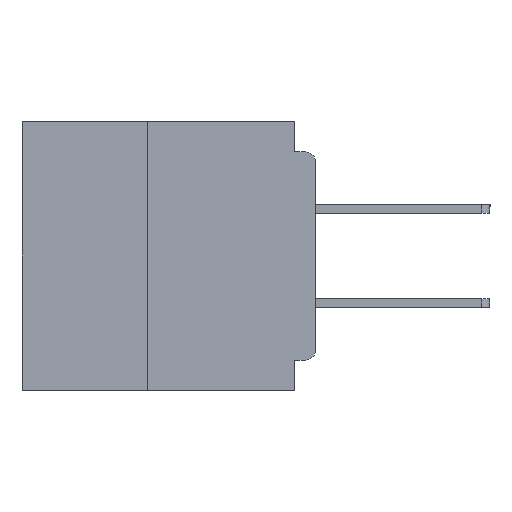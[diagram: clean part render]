
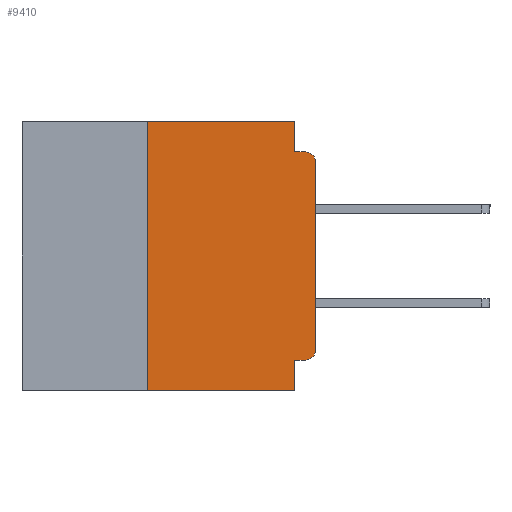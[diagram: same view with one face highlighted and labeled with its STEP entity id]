
A CAD part, left-side view. The second image highlights one B-rep face of the part: STEP entity #9410.
In plain terms, the highlighted planar face has unit normal (-1, 0, 0).
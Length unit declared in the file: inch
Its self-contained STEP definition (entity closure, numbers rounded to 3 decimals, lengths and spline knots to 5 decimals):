
#343 = VECTOR ( 'NONE', #35084, 39.37008 ) ;
#1396 = VECTOR ( 'NONE', #38408, 39.37008 ) ;
#1498 = VERTEX_POINT ( 'NONE', #6303 ) ;
#2432 = DIRECTION ( 'NONE',  ( 0., 0., -1. ) ) ;
#2590 = CARTESIAN_POINT ( 'NONE',  ( 0., 0.437, 0. ) ) ;
#2696 = EDGE_CURVE ( 'NONE', #32461, #8480, #12332, .T. ) ;
#3576 = CARTESIAN_POINT ( 'NONE',  ( 0., 0.031, 0. ) ) ;
#3684 = CARTESIAN_POINT ( 'NONE',  ( 0., 0.015, -0.06 ) ) ;
#4846 = CARTESIAN_POINT ( 'NONE',  ( 0., 0.437, -0.4 ) ) ;
#5216 = ORIENTED_EDGE ( 'NONE', *, *, #17932, .F. ) ;
#5430 = EDGE_CURVE ( 'NONE', #10705, #7421, #14539, .T. ) ;
#5847 = DIRECTION ( 'NONE',  ( 0., -1., 0. ) ) ;
#6114 = CARTESIAN_POINT ( 'NONE',  ( 0., 0.031, -0.4 ) ) ;
#6303 = CARTESIAN_POINT ( 'NONE',  ( 0., 0.25, -0.4 ) ) ;
#6957 = DIRECTION ( 'NONE',  ( 0., 0., -1. ) ) ;
#7421 = VERTEX_POINT ( 'NONE', #6114 ) ;
#7553 = CIRCLE ( 'NONE', #32367, 0.015 ) ;
#7854 = CARTESIAN_POINT ( 'NONE',  ( 0., 0.031, -0.045 ) ) ;
#8061 = CARTESIAN_POINT ( 'NONE',  ( 0., 0., -0.34 ) ) ;
#8124 = DIRECTION ( 'NONE',  ( 0., -1., 0. ) ) ;
#8434 = CARTESIAN_POINT ( 'NONE',  ( 0., 0.015, -0.34 ) ) ;
#8480 = VERTEX_POINT ( 'NONE', #8061 ) ;
#8983 = VECTOR ( 'NONE', #5847, 39.37008 ) ;
#9410 = ADVANCED_FACE ( 'NONE', ( #22653 ), #12601, .F. ) ;
#10026 = LINE ( 'NONE', #38281, #1396 ) ;
#10174 = VECTOR ( 'NONE', #24136, 39.37008 ) ;
#10698 = EDGE_CURVE ( 'NONE', #32712, #36361, #7553, .T. ) ;
#10705 = VERTEX_POINT ( 'NONE', #35441 ) ;
#11153 = LINE ( 'NONE', #39846, #10174 ) ;
#11665 = DIRECTION ( 'NONE',  ( 0., 0., -1. ) ) ;
#12332 = CIRCLE ( 'NONE', #27303, 0.015 ) ;
#12601 = PLANE ( 'NONE',  #35552 ) ;
#13290 = CARTESIAN_POINT ( 'NONE',  ( 0., 0.25, 0. ) ) ;
#14539 = LINE ( 'NONE', #37370, #37810 ) ;
#14690 = ORIENTED_EDGE ( 'NONE', *, *, #39548, .T. ) ;
#16195 = EDGE_CURVE ( 'NONE', #1498, #40842, #11153, .T. ) ;
#16479 = ORIENTED_EDGE ( 'NONE', *, *, #2696, .T. ) ;
#17708 = VERTEX_POINT ( 'NONE', #7854 ) ;
#17932 = EDGE_CURVE ( 'NONE', #40842, #19446, #34314, .T. ) ;
#18294 = CARTESIAN_POINT ( 'NONE',  ( 0., 0., -0.06 ) ) ;
#19059 = EDGE_CURVE ( 'NONE', #19446, #17708, #25350, .T. ) ;
#19446 = VERTEX_POINT ( 'NONE', #3576 ) ;
#19462 = CARTESIAN_POINT ( 'NONE',  ( 0., 0.015, -0.045 ) ) ;
#19996 = CARTESIAN_POINT ( 'NONE',  ( 0., 0.015, -0.355 ) ) ;
#20635 = CARTESIAN_POINT ( 'NONE',  ( 0., 0., 0. ) ) ;
#21001 = ORIENTED_EDGE ( 'NONE', *, *, #33848, .F. ) ;
#21851 = ORIENTED_EDGE ( 'NONE', *, *, #5430, .F. ) ;
#22653 = FACE_OUTER_BOUND ( 'NONE', #26862, .T. ) ;
#22950 = EDGE_CURVE ( 'NONE', #8480, #32712, #36815, .T. ) ;
#24136 = DIRECTION ( 'NONE',  ( 0., 0., 1. ) ) ;
#24366 = CARTESIAN_POINT ( 'NONE',  ( 0., 0.031, 0. ) ) ;
#25283 = DIRECTION ( 'NONE',  ( 1., 0., 0. ) ) ;
#25350 = LINE ( 'NONE', #24366, #32699 ) ;
#26053 = DIRECTION ( 'NONE',  ( -1., 0., 0. ) ) ;
#26862 = EDGE_LOOP ( 'NONE', ( #41240, #37259, #21001, #28418, #5216, #30133, #14690, #21851, #36398, #16479 ) ) ;
#26868 = LINE ( 'NONE', #31880, #343 ) ;
#26954 = DIRECTION ( 'NONE',  ( 0., 0., 1. ) ) ;
#27303 = AXIS2_PLACEMENT_3D ( 'NONE', #8434, #30661, #11665 ) ;
#28418 = ORIENTED_EDGE ( 'NONE', *, *, #19059, .F. ) ;
#28427 = CARTESIAN_POINT ( 'NONE',  ( 0., 0.437, 0. ) ) ;
#30133 = ORIENTED_EDGE ( 'NONE', *, *, #16195, .F. ) ;
#30661 = DIRECTION ( 'NONE',  ( -1., 0., 0. ) ) ;
#31880 = CARTESIAN_POINT ( 'NONE',  ( 0., 0., -0.355 ) ) ;
#32367 = AXIS2_PLACEMENT_3D ( 'NONE', #3684, #26053, #6957 ) ;
#32461 = VERTEX_POINT ( 'NONE', #19996 ) ;
#32490 = VECTOR ( 'NONE', #8124, 39.37008 ) ;
#32699 = VECTOR ( 'NONE', #33858, 39.37008 ) ;
#32712 = VERTEX_POINT ( 'NONE', #18294 ) ;
#33848 = EDGE_CURVE ( 'NONE', #17708, #36361, #10026, .T. ) ;
#33858 = DIRECTION ( 'NONE',  ( 0., 0., -1. ) ) ;
#34314 = LINE ( 'NONE', #2590, #8983 ) ;
#34789 = DIRECTION ( 'NONE',  ( 0., 0., -1. ) ) ;
#35084 = DIRECTION ( 'NONE',  ( 0., 1., 0. ) ) ;
#35441 = CARTESIAN_POINT ( 'NONE',  ( 0., 0.031, -0.355 ) ) ;
#35552 = AXIS2_PLACEMENT_3D ( 'NONE', #28427, #25283, #34789 ) ;
#35825 = VECTOR ( 'NONE', #26954, 39.37008 ) ;
#36313 = EDGE_CURVE ( 'NONE', #32461, #10705, #26868, .T. ) ;
#36361 = VERTEX_POINT ( 'NONE', #19462 ) ;
#36398 = ORIENTED_EDGE ( 'NONE', *, *, #36313, .F. ) ;
#36815 = LINE ( 'NONE', #20635, #35825 ) ;
#37259 = ORIENTED_EDGE ( 'NONE', *, *, #10698, .T. ) ;
#37370 = CARTESIAN_POINT ( 'NONE',  ( 0., 0.031, -0.4 ) ) ;
#37810 = VECTOR ( 'NONE', #2432, 39.37008 ) ;
#38281 = CARTESIAN_POINT ( 'NONE',  ( 0., 0., -0.045 ) ) ;
#38408 = DIRECTION ( 'NONE',  ( 0., -1., 0. ) ) ;
#39548 = EDGE_CURVE ( 'NONE', #1498, #7421, #40896, .T. ) ;
#39846 = CARTESIAN_POINT ( 'NONE',  ( 0., 0.25, -0.4 ) ) ;
#40842 = VERTEX_POINT ( 'NONE', #13290 ) ;
#40896 = LINE ( 'NONE', #4846, #32490 ) ;
#41240 = ORIENTED_EDGE ( 'NONE', *, *, #22950, .T. ) ;
